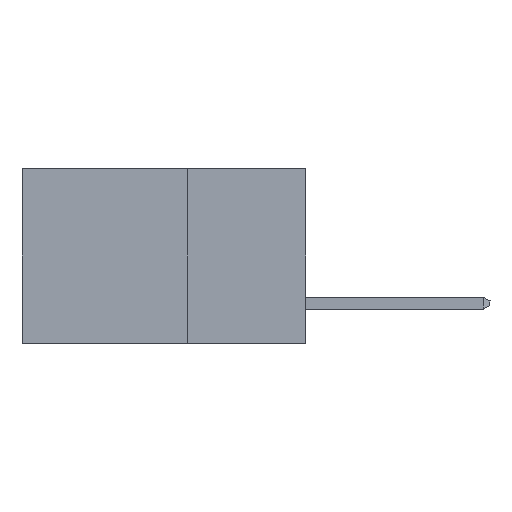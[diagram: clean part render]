
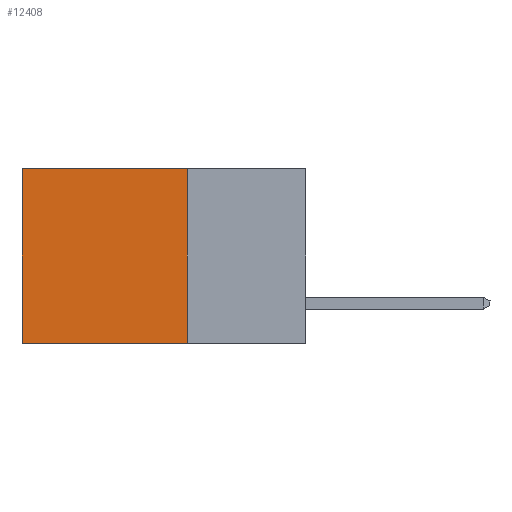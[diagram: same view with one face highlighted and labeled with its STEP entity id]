
A CAD part, left-side view. The second image highlights one B-rep face of the part: STEP entity #12408.
In plain terms, the highlighted planar face has unit normal (-1, 0, 0).
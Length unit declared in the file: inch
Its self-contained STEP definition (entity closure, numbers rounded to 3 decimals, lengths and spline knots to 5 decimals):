
#20 = VERTEX_POINT ( 'NONE', #5017 ) ;
#339 = EDGE_CURVE ( 'NONE', #12559, #457, #11381, .T. ) ;
#457 = VERTEX_POINT ( 'NONE', #6828 ) ;
#681 = VECTOR ( 'NONE', #5575, 39.37008 ) ;
#1038 = ORIENTED_EDGE ( 'NONE', *, *, #6690, .T. ) ;
#1812 = LINE ( 'NONE', #3316, #9076 ) ;
#2144 = DIRECTION ( 'NONE',  ( 0., 0., -1. ) ) ;
#3178 = DIRECTION ( 'NONE',  ( 1., 0., 0. ) ) ;
#3186 = CARTESIAN_POINT ( 'NONE',  ( 0.298, 0.25, -0.37 ) ) ;
#3316 = CARTESIAN_POINT ( 'NONE',  ( 0.298, 0.25, 0. ) ) ;
#4425 = ORIENTED_EDGE ( 'NONE', *, *, #7978, .F. ) ;
#4648 = CARTESIAN_POINT ( 'NONE',  ( 0.298, 0.6, 0. ) ) ;
#5017 = CARTESIAN_POINT ( 'NONE',  ( 0.298, 0.25, 0. ) ) ;
#5575 = DIRECTION ( 'NONE',  ( 0., 1., 0. ) ) ;
#6135 = FACE_OUTER_BOUND ( 'NONE', #13836, .T. ) ;
#6607 = VECTOR ( 'NONE', #6628, 39.37008 ) ;
#6628 = DIRECTION ( 'NONE',  ( 0., 0., -1. ) ) ;
#6690 = EDGE_CURVE ( 'NONE', #20, #12559, #10729, .T. ) ;
#6767 = DIRECTION ( 'NONE',  ( 0., 0., -1. ) ) ;
#6823 = ORIENTED_EDGE ( 'NONE', *, *, #339, .T. ) ;
#6828 = CARTESIAN_POINT ( 'NONE',  ( 0.298, 0.6, -0.37 ) ) ;
#7722 = VECTOR ( 'NONE', #12254, 39.37008 ) ;
#7978 = EDGE_CURVE ( 'NONE', #20, #8938, #1812, .T. ) ;
#8938 = VERTEX_POINT ( 'NONE', #10183 ) ;
#9076 = VECTOR ( 'NONE', #6767, 39.37008 ) ;
#10183 = CARTESIAN_POINT ( 'NONE',  ( 0.298, 0.25, -0.37 ) ) ;
#10729 = LINE ( 'NONE', #13466, #7722 ) ;
#11128 = CARTESIAN_POINT ( 'NONE',  ( 0.298, 0.25, 0. ) ) ;
#11136 = CARTESIAN_POINT ( 'NONE',  ( 0.298, 0.6, 0. ) ) ;
#11219 = EDGE_CURVE ( 'NONE', #8938, #457, #11478, .T. ) ;
#11277 = AXIS2_PLACEMENT_3D ( 'NONE', #11128, #3178, #2144 ) ;
#11381 = LINE ( 'NONE', #11136, #6607 ) ;
#11478 = LINE ( 'NONE', #3186, #681 ) ;
#11782 = ORIENTED_EDGE ( 'NONE', *, *, #11219, .F. ) ;
#12254 = DIRECTION ( 'NONE',  ( 0., 1., 0. ) ) ;
#12408 = ADVANCED_FACE ( 'NONE', ( #6135 ), #14459, .F. ) ;
#12559 = VERTEX_POINT ( 'NONE', #4648 ) ;
#13466 = CARTESIAN_POINT ( 'NONE',  ( 0.298, 0.25, 0. ) ) ;
#13836 = EDGE_LOOP ( 'NONE', ( #6823, #11782, #4425, #1038 ) ) ;
#14459 = PLANE ( 'NONE',  #11277 ) ;
